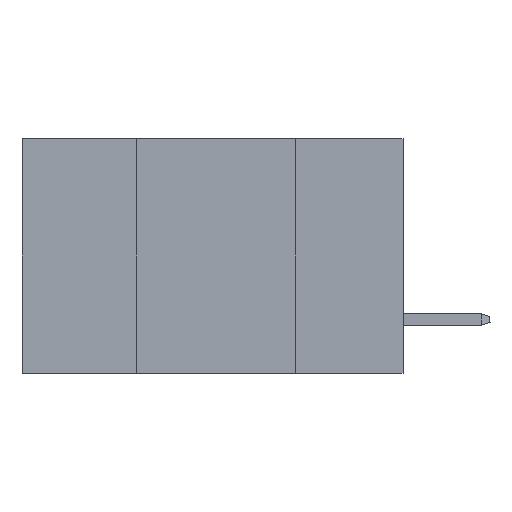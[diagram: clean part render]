
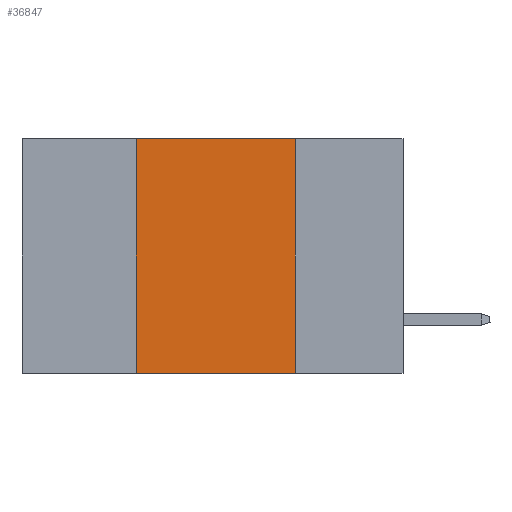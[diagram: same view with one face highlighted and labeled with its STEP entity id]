
A CAD part, left-side view. The second image highlights one B-rep face of the part: STEP entity #36847.
In plain terms, the highlighted planar face has unit normal (-1, 0, 0).
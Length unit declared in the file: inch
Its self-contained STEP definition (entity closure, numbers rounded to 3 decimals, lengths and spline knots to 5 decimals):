
#1595 = EDGE_LOOP ( 'NONE', ( #16092, #29561, #24373, #20586 ) ) ;
#3393 = DIRECTION ( 'NONE',  ( 0., -1., 0. ) ) ;
#4149 = VECTOR ( 'NONE', #21291, 39.37008 ) ;
#5525 = CARTESIAN_POINT ( 'NONE',  ( 0., 0.17, 0. ) ) ;
#6791 = LINE ( 'NONE', #9257, #25660 ) ;
#7043 = CARTESIAN_POINT ( 'NONE',  ( 0., 0.42, 0. ) ) ;
#7989 = LINE ( 'NONE', #5525, #20884 ) ;
#9257 = CARTESIAN_POINT ( 'NONE',  ( 0., 0.6, 0. ) ) ;
#10631 = VERTEX_POINT ( 'NONE', #35395 ) ;
#11113 = CARTESIAN_POINT ( 'NONE',  ( 0., 0.17, -0.37 ) ) ;
#11541 = VECTOR ( 'NONE', #24032, 39.37008 ) ;
#12908 = LINE ( 'NONE', #7043, #11541 ) ;
#15762 = DIRECTION ( 'NONE',  ( 1., 0., 0. ) ) ;
#16092 = ORIENTED_EDGE ( 'NONE', *, *, #22411, .F. ) ;
#18464 = CARTESIAN_POINT ( 'NONE',  ( 0., 0.6, -0.37 ) ) ;
#18775 = FACE_OUTER_BOUND ( 'NONE', #1595, .T. ) ;
#20586 = ORIENTED_EDGE ( 'NONE', *, *, #27686, .T. ) ;
#20884 = VECTOR ( 'NONE', #28373, 39.37008 ) ;
#21291 = DIRECTION ( 'NONE',  ( 0., -1., 0. ) ) ;
#21350 = CARTESIAN_POINT ( 'NONE',  ( 0., 0.42, -0.37 ) ) ;
#21789 = EDGE_CURVE ( 'NONE', #26719, #10631, #6791, .T. ) ;
#22411 = EDGE_CURVE ( 'NONE', #10631, #25830, #7989, .T. ) ;
#24032 = DIRECTION ( 'NONE',  ( 0., 0., 1. ) ) ;
#24373 = ORIENTED_EDGE ( 'NONE', *, *, #29927, .F. ) ;
#25660 = VECTOR ( 'NONE', #3393, 39.37008 ) ;
#25830 = VERTEX_POINT ( 'NONE', #11113 ) ;
#26719 = VERTEX_POINT ( 'NONE', #31920 ) ;
#27686 = EDGE_CURVE ( 'NONE', #30314, #25830, #35839, .T. ) ;
#28373 = DIRECTION ( 'NONE',  ( 0., 0., -1. ) ) ;
#29561 = ORIENTED_EDGE ( 'NONE', *, *, #21789, .F. ) ;
#29927 = EDGE_CURVE ( 'NONE', #30314, #26719, #12908, .T. ) ;
#30288 = PLANE ( 'NONE',  #36412 ) ;
#30314 = VERTEX_POINT ( 'NONE', #21350 ) ;
#31920 = CARTESIAN_POINT ( 'NONE',  ( 0., 0.42, 0. ) ) ;
#33315 = DIRECTION ( 'NONE',  ( 0., 0., -1. ) ) ;
#35395 = CARTESIAN_POINT ( 'NONE',  ( 0., 0.17, 0. ) ) ;
#35839 = LINE ( 'NONE', #18464, #4149 ) ;
#35979 = CARTESIAN_POINT ( 'NONE',  ( 0., 0.6, 0. ) ) ;
#36412 = AXIS2_PLACEMENT_3D ( 'NONE', #35979, #15762, #33315 ) ;
#36847 = ADVANCED_FACE ( 'NONE', ( #18775 ), #30288, .F. ) ;
